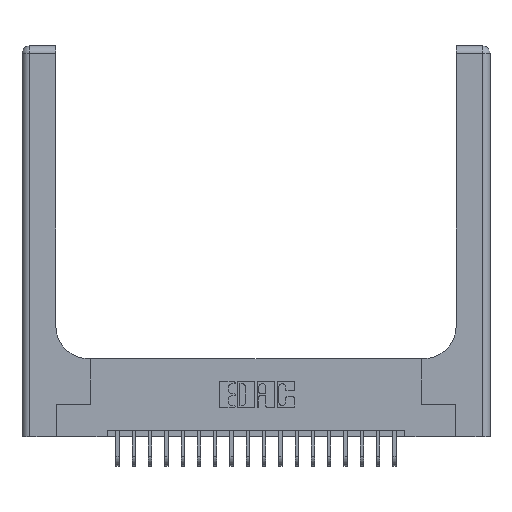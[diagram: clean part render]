
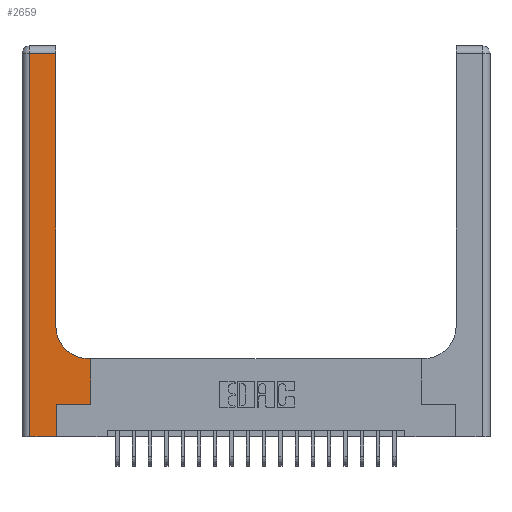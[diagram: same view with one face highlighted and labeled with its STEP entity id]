
A CAD part, top view. The second image highlights one B-rep face of the part: STEP entity #2659.
In plain terms, the highlighted planar face has unit normal (0, 0, 1).
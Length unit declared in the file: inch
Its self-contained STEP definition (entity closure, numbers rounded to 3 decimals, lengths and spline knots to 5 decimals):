
#541 = EDGE_CURVE ( 'NONE', #19493, #4466, #3964, .T. ) ;
#599 = ORIENTED_EDGE ( 'NONE', *, *, #16676, .T. ) ;
#693 = ORIENTED_EDGE ( 'NONE', *, *, #9551, .T. ) ;
#774 = EDGE_LOOP ( 'NONE', ( #21773, #599, #693, #13945, #21155, #19390, #21728, #18213, #2580 ) ) ;
#909 = CARTESIAN_POINT ( 'NONE',  ( 0., 2.94, 0.37 ) ) ;
#993 = VECTOR ( 'NONE', #21825, 39.37008 ) ;
#1086 = CARTESIAN_POINT ( 'NONE',  ( 0.528, 0.25, 0.37 ) ) ;
#1383 = LINE ( 'NONE', #7150, #5334 ) ;
#1790 = VECTOR ( 'NONE', #8271, 39.37008 ) ;
#1999 = AXIS2_PLACEMENT_3D ( 'NONE', #10632, #14051, #17608 ) ;
#2026 = CARTESIAN_POINT ( 'NONE',  ( 0.06, 3., 0.37 ) ) ;
#2321 = CARTESIAN_POINT ( 'NONE',  ( 0.265, 0.25, 0.37 ) ) ;
#2580 = ORIENTED_EDGE ( 'NONE', *, *, #11905, .T. ) ;
#2640 = CARTESIAN_POINT ( 'NONE',  ( 0.528, 0.6, 0.37 ) ) ;
#2659 = ADVANCED_FACE ( 'NONE', ( #17132 ), #15634, .F. ) ;
#2894 = VERTEX_POINT ( 'NONE', #2640 ) ;
#3358 = DIRECTION ( 'NONE',  ( 1., 0., 0. ) ) ;
#3529 = DIRECTION ( 'NONE',  ( 0., -1., 0. ) ) ;
#3716 = DIRECTION ( 'NONE',  ( 1., 0., 0. ) ) ;
#3767 = VECTOR ( 'NONE', #3529, 39.37008 ) ;
#3775 = VERTEX_POINT ( 'NONE', #16281 ) ;
#3964 = LINE ( 'NONE', #9493, #21506 ) ;
#4466 = VERTEX_POINT ( 'NONE', #10954 ) ;
#5063 = LINE ( 'NONE', #2026, #3767 ) ;
#5334 = VECTOR ( 'NONE', #13755, 39.37008 ) ;
#5348 = EDGE_CURVE ( 'NONE', #7192, #3775, #14694, .T. ) ;
#5350 = DIRECTION ( 'NONE',  ( 0., 0., -1. ) ) ;
#5482 = LINE ( 'NONE', #11438, #993 ) ;
#6577 = CARTESIAN_POINT ( 'NONE',  ( 0.265, 0., 0.37 ) ) ;
#7150 = CARTESIAN_POINT ( 'NONE',  ( 0.528, 0.25, 0.37 ) ) ;
#7192 = VERTEX_POINT ( 'NONE', #12774 ) ;
#7627 = LINE ( 'NONE', #6577, #1790 ) ;
#8271 = DIRECTION ( 'NONE',  ( 0., 1., 0. ) ) ;
#8326 = CARTESIAN_POINT ( 'NONE',  ( 0., 0., 0.37 ) ) ;
#8584 = VECTOR ( 'NONE', #21169, 39.37008 ) ;
#8610 = CARTESIAN_POINT ( 'NONE',  ( 0.51, 0.6, 0.37 ) ) ;
#9493 = CARTESIAN_POINT ( 'NONE',  ( 0.26, 3., 0.37 ) ) ;
#9551 = EDGE_CURVE ( 'NONE', #14098, #7192, #5063, .T. ) ;
#9673 = VECTOR ( 'NONE', #3358, 39.37008 ) ;
#9771 = AXIS2_PLACEMENT_3D ( 'NONE', #11981, #5350, #10491 ) ;
#10277 = EDGE_CURVE ( 'NONE', #12451, #21410, #21267, .T. ) ;
#10491 = DIRECTION ( 'NONE',  ( -1., 0., 0. ) ) ;
#10632 = CARTESIAN_POINT ( 'NONE',  ( 0.51, 0.85, 0.37 ) ) ;
#10954 = CARTESIAN_POINT ( 'NONE',  ( 0.26, 2.94, 0.37 ) ) ;
#11438 = CARTESIAN_POINT ( 'NONE',  ( 0.26, 0.6, 0.37 ) ) ;
#11905 = EDGE_CURVE ( 'NONE', #12825, #19493, #20661, .T. ) ;
#11981 = CARTESIAN_POINT ( 'NONE',  ( 0., 3., 0.37 ) ) ;
#12451 = VERTEX_POINT ( 'NONE', #2321 ) ;
#12662 = EDGE_CURVE ( 'NONE', #2894, #12825, #5482, .T. ) ;
#12774 = CARTESIAN_POINT ( 'NONE',  ( 0.06, 0., 0.37 ) ) ;
#12825 = VERTEX_POINT ( 'NONE', #8610 ) ;
#13040 = VECTOR ( 'NONE', #3716, 39.37008 ) ;
#13755 = DIRECTION ( 'NONE',  ( 0., 1., 0. ) ) ;
#13864 = CARTESIAN_POINT ( 'NONE',  ( 0.265, 0.25, 0.37 ) ) ;
#13945 = ORIENTED_EDGE ( 'NONE', *, *, #5348, .T. ) ;
#14051 = DIRECTION ( 'NONE',  ( 0., 0., -1. ) ) ;
#14098 = VERTEX_POINT ( 'NONE', #18494 ) ;
#14694 = LINE ( 'NONE', #8326, #9673 ) ;
#15108 = DIRECTION ( 'NONE',  ( 0., 1., 0. ) ) ;
#15634 = PLANE ( 'NONE',  #9771 ) ;
#16281 = CARTESIAN_POINT ( 'NONE',  ( 0.265, 0., 0.37 ) ) ;
#16520 = CARTESIAN_POINT ( 'NONE',  ( 0.26, 0.85, 0.37 ) ) ;
#16676 = EDGE_CURVE ( 'NONE', #4466, #14098, #18654, .T. ) ;
#17132 = FACE_OUTER_BOUND ( 'NONE', #774, .T. ) ;
#17422 = EDGE_CURVE ( 'NONE', #21410, #2894, #1383, .T. ) ;
#17608 = DIRECTION ( 'NONE',  ( 1., 0., 0. ) ) ;
#18213 = ORIENTED_EDGE ( 'NONE', *, *, #12662, .T. ) ;
#18494 = CARTESIAN_POINT ( 'NONE',  ( 0.06, 2.94, 0.37 ) ) ;
#18654 = LINE ( 'NONE', #909, #8584 ) ;
#19390 = ORIENTED_EDGE ( 'NONE', *, *, #10277, .T. ) ;
#19493 = VERTEX_POINT ( 'NONE', #16520 ) ;
#20661 = CIRCLE ( 'NONE', #1999, 0.25 ) ;
#21155 = ORIENTED_EDGE ( 'NONE', *, *, #21668, .T. ) ;
#21169 = DIRECTION ( 'NONE',  ( -1., 0., 0. ) ) ;
#21267 = LINE ( 'NONE', #13864, #13040 ) ;
#21410 = VERTEX_POINT ( 'NONE', #1086 ) ;
#21506 = VECTOR ( 'NONE', #15108, 39.37008 ) ;
#21668 = EDGE_CURVE ( 'NONE', #3775, #12451, #7627, .T. ) ;
#21728 = ORIENTED_EDGE ( 'NONE', *, *, #17422, .T. ) ;
#21773 = ORIENTED_EDGE ( 'NONE', *, *, #541, .T. ) ;
#21825 = DIRECTION ( 'NONE',  ( -1., 0., 0. ) ) ;
